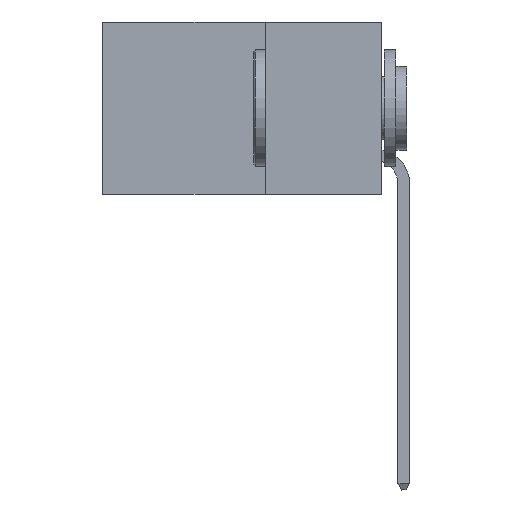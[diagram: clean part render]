
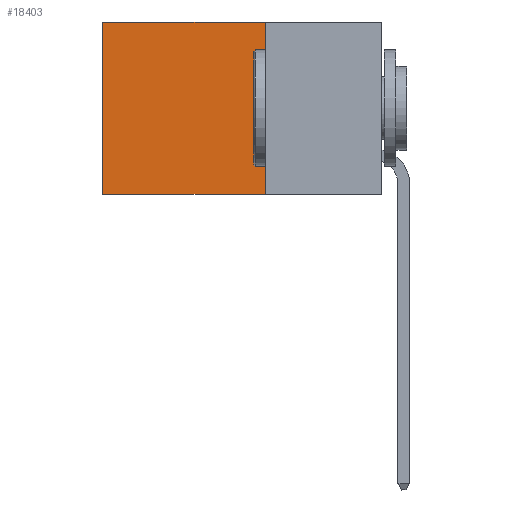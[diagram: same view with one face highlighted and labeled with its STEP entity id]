
A CAD part, left-side view. The second image highlights one B-rep face of the part: STEP entity #18403.
In plain terms, the highlighted planar face has unit normal (-1, 0, 0).
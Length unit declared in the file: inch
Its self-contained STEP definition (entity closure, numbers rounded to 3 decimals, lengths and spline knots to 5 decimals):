
#346 = CARTESIAN_POINT ( 'NONE',  ( 0.2875, 0.6, -0.37 ) ) ;
#901 = LINE ( 'NONE', #29146, #50643 ) ;
#1231 = DIRECTION ( 'NONE',  ( 0., 0., -1. ) ) ;
#1739 = DIRECTION ( 'NONE',  ( 0., 1., 0. ) ) ;
#2548 = LINE ( 'NONE', #33032, #9265 ) ;
#2971 = VERTEX_POINT ( 'NONE', #25332 ) ;
#5693 = ORIENTED_EDGE ( 'NONE', *, *, #36123, .F. ) ;
#9265 = VECTOR ( 'NONE', #1739, 39.37008 ) ;
#10597 = AXIS2_PLACEMENT_3D ( 'NONE', #40272, #40437, #1231 ) ;
#13239 = EDGE_LOOP ( 'NONE', ( #15825, #47223, #5693, #26095 ) ) ;
#13887 = DIRECTION ( 'NONE',  ( 0., 0., -1. ) ) ;
#14740 = VERTEX_POINT ( 'NONE', #42492 ) ;
#15825 = ORIENTED_EDGE ( 'NONE', *, *, #45233, .T. ) ;
#17690 = CARTESIAN_POINT ( 'NONE',  ( 0.2875, 0.25, 0. ) ) ;
#18403 = ADVANCED_FACE ( 'NONE', ( #29757 ), #36127, .F. ) ;
#19984 = EDGE_CURVE ( 'NONE', #2971, #14740, #2548, .T. ) ;
#21583 = VERTEX_POINT ( 'NONE', #346 ) ;
#25332 = CARTESIAN_POINT ( 'NONE',  ( 0.2875, 0.25, 0. ) ) ;
#26095 = ORIENTED_EDGE ( 'NONE', *, *, #19984, .T. ) ;
#28635 = CARTESIAN_POINT ( 'NONE',  ( 0.2875, 0.6, 0. ) ) ;
#29146 = CARTESIAN_POINT ( 'NONE',  ( 0.2875, 0.25, -0.37 ) ) ;
#29482 = VECTOR ( 'NONE', #13887, 39.37008 ) ;
#29757 = FACE_OUTER_BOUND ( 'NONE', #13239, .T. ) ;
#31039 = LINE ( 'NONE', #28635, #45782 ) ;
#33032 = CARTESIAN_POINT ( 'NONE',  ( 0.2875, 0.25, 0. ) ) ;
#36123 = EDGE_CURVE ( 'NONE', #2971, #37934, #41169, .T. ) ;
#36127 = PLANE ( 'NONE',  #10597 ) ;
#37934 = VERTEX_POINT ( 'NONE', #39037 ) ;
#39037 = CARTESIAN_POINT ( 'NONE',  ( 0.2875, 0.25, -0.37 ) ) ;
#40272 = CARTESIAN_POINT ( 'NONE',  ( 0.2875, 0.25, 0. ) ) ;
#40306 = DIRECTION ( 'NONE',  ( 0., 1., 0. ) ) ;
#40437 = DIRECTION ( 'NONE',  ( 1., 0., 0. ) ) ;
#41169 = LINE ( 'NONE', #17690, #29482 ) ;
#42492 = CARTESIAN_POINT ( 'NONE',  ( 0.2875, 0.6, 0. ) ) ;
#44421 = DIRECTION ( 'NONE',  ( 0., 0., -1. ) ) ;
#45233 = EDGE_CURVE ( 'NONE', #14740, #21583, #31039, .T. ) ;
#45778 = EDGE_CURVE ( 'NONE', #37934, #21583, #901, .T. ) ;
#45782 = VECTOR ( 'NONE', #44421, 39.37008 ) ;
#47223 = ORIENTED_EDGE ( 'NONE', *, *, #45778, .F. ) ;
#50643 = VECTOR ( 'NONE', #40306, 39.37008 ) ;
